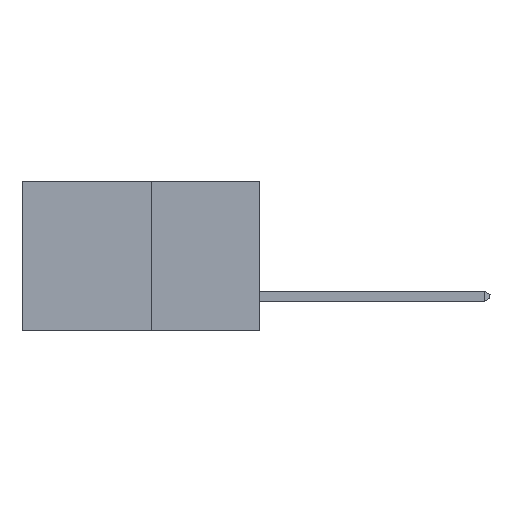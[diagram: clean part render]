
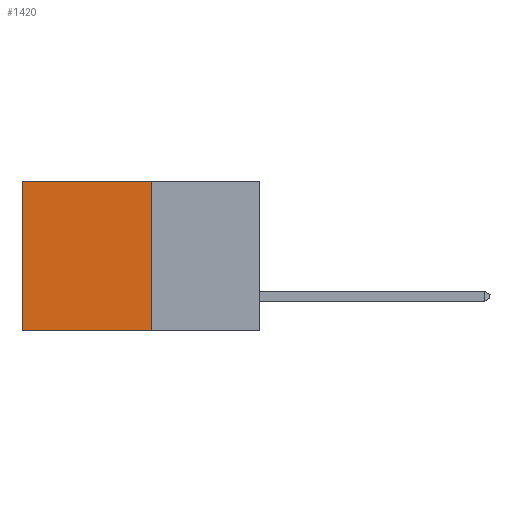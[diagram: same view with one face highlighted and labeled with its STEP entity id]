
A CAD part, left-side view. The second image highlights one B-rep face of the part: STEP entity #1420.
In plain terms, the highlighted planar face has unit normal (-1, 0, 0).
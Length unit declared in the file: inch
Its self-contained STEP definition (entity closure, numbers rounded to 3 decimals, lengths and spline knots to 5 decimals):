
#309 = EDGE_LOOP ( 'NONE', ( #4444, #3921, #1910, #8048 ) ) ;
#409 = DIRECTION ( 'NONE',  ( 1., 0., 0. ) ) ;
#1420 = ADVANCED_FACE ( 'NONE', ( #1989 ), #8099, .F. ) ;
#1642 = VERTEX_POINT ( 'NONE', #8222 ) ;
#1910 = ORIENTED_EDGE ( 'NONE', *, *, #3387, .F. ) ;
#1989 = FACE_OUTER_BOUND ( 'NONE', #309, .T. ) ;
#2309 = VERTEX_POINT ( 'NONE', #5032 ) ;
#3387 = EDGE_CURVE ( 'NONE', #2309, #9844, #4883, .T. ) ;
#3921 = ORIENTED_EDGE ( 'NONE', *, *, #5326, .F. ) ;
#3940 = EDGE_CURVE ( 'NONE', #1642, #4154, #10042, .T. ) ;
#4119 = VECTOR ( 'NONE', #8338, 39.37008 ) ;
#4154 = VERTEX_POINT ( 'NONE', #8491 ) ;
#4234 = VECTOR ( 'NONE', #9209, 39.37008 ) ;
#4311 = CARTESIAN_POINT ( 'NONE',  ( 0.277, 0.27, -0.37 ) ) ;
#4444 = ORIENTED_EDGE ( 'NONE', *, *, #3940, .T. ) ;
#4631 = VECTOR ( 'NONE', #5465, 39.37008 ) ;
#4639 = EDGE_CURVE ( 'NONE', #2309, #1642, #10131, .T. ) ;
#4883 = LINE ( 'NONE', #5848, #4631 ) ;
#5032 = CARTESIAN_POINT ( 'NONE',  ( 0.277, 0.27, 0. ) ) ;
#5326 = EDGE_CURVE ( 'NONE', #9844, #4154, #7977, .T. ) ;
#5465 = DIRECTION ( 'NONE',  ( 0., 0., -1. ) ) ;
#5848 = CARTESIAN_POINT ( 'NONE',  ( 0.277, 0.27, -0.37 ) ) ;
#6466 = DIRECTION ( 'NONE',  ( 0., 0., -1. ) ) ;
#7268 = AXIS2_PLACEMENT_3D ( 'NONE', #4311, #409, #6466 ) ;
#7734 = VECTOR ( 'NONE', #9108, 39.37008 ) ;
#7755 = CARTESIAN_POINT ( 'NONE',  ( 0.277, 0.59, -0.37 ) ) ;
#7977 = LINE ( 'NONE', #9539, #7734 ) ;
#8048 = ORIENTED_EDGE ( 'NONE', *, *, #4639, .T. ) ;
#8099 = PLANE ( 'NONE',  #7268 ) ;
#8160 = CARTESIAN_POINT ( 'NONE',  ( 0.277, 0.27, -0.37 ) ) ;
#8222 = CARTESIAN_POINT ( 'NONE',  ( 0.277, 0.59, 0. ) ) ;
#8338 = DIRECTION ( 'NONE',  ( 0., 0., -1. ) ) ;
#8491 = CARTESIAN_POINT ( 'NONE',  ( 0.277, 0.59, -0.37 ) ) ;
#9108 = DIRECTION ( 'NONE',  ( 0., 1., 0. ) ) ;
#9209 = DIRECTION ( 'NONE',  ( 0., 1., 0. ) ) ;
#9503 = CARTESIAN_POINT ( 'NONE',  ( 0.277, 0.27, 0. ) ) ;
#9539 = CARTESIAN_POINT ( 'NONE',  ( 0.277, 0.27, -0.37 ) ) ;
#9844 = VERTEX_POINT ( 'NONE', #8160 ) ;
#10042 = LINE ( 'NONE', #7755, #4119 ) ;
#10131 = LINE ( 'NONE', #9503, #4234 ) ;
